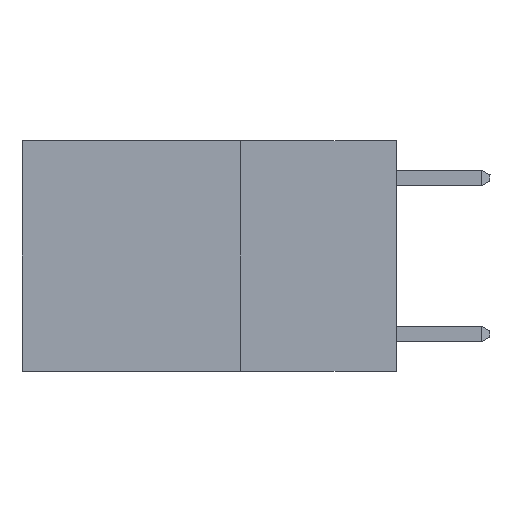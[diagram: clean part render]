
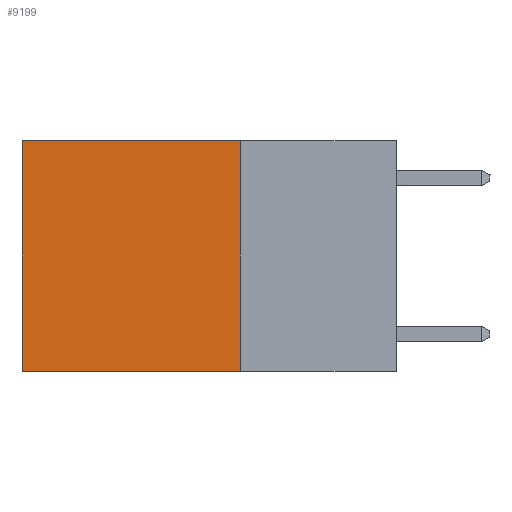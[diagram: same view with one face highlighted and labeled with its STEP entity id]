
A CAD part, left-side view. The second image highlights one B-rep face of the part: STEP entity #9199.
In plain terms, the highlighted planar face has unit normal (-1, 0, 0).
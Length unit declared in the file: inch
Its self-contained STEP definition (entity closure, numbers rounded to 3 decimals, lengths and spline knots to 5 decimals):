
#238 = VERTEX_POINT ( 'NONE', #22340 ) ;
#994 = VERTEX_POINT ( 'NONE', #19007 ) ;
#1125 = LINE ( 'NONE', #6130, #4509 ) ;
#1518 = VECTOR ( 'NONE', #5088, 39.37008 ) ;
#1844 = CARTESIAN_POINT ( 'NONE',  ( 0.2625, 0.6, 0. ) ) ;
#3830 = PLANE ( 'NONE',  #23399 ) ;
#4509 = VECTOR ( 'NONE', #24514, 39.37008 ) ;
#5088 = DIRECTION ( 'NONE',  ( 0., 0., -1. ) ) ;
#5142 = ORIENTED_EDGE ( 'NONE', *, *, #10766, .T. ) ;
#6130 = CARTESIAN_POINT ( 'NONE',  ( 0.2625, 0.25, -0.37 ) ) ;
#8123 = EDGE_LOOP ( 'NONE', ( #5142, #9700, #16774, #9651 ) ) ;
#9199 = ADVANCED_FACE ( 'NONE', ( #30511 ), #3830, .F. ) ;
#9651 = ORIENTED_EDGE ( 'NONE', *, *, #12834, .T. ) ;
#9700 = ORIENTED_EDGE ( 'NONE', *, *, #12046, .F. ) ;
#10766 = EDGE_CURVE ( 'NONE', #20575, #18777, #12174, .T. ) ;
#11542 = CARTESIAN_POINT ( 'NONE',  ( 0.2625, 0.25, 0. ) ) ;
#11650 = CARTESIAN_POINT ( 'NONE',  ( 0.2625, 0.6, 0. ) ) ;
#12046 = EDGE_CURVE ( 'NONE', #994, #18777, #1125, .T. ) ;
#12174 = LINE ( 'NONE', #1844, #23972 ) ;
#12830 = EDGE_CURVE ( 'NONE', #238, #994, #21905, .T. ) ;
#12834 = EDGE_CURVE ( 'NONE', #238, #20575, #16902, .T. ) ;
#13761 = DIRECTION ( 'NONE',  ( 1., 0., 0. ) ) ;
#14233 = CARTESIAN_POINT ( 'NONE',  ( 0.2625, 0.6, -0.37 ) ) ;
#14701 = DIRECTION ( 'NONE',  ( 0., 1., 0. ) ) ;
#16774 = ORIENTED_EDGE ( 'NONE', *, *, #12830, .F. ) ;
#16902 = LINE ( 'NONE', #17051, #24580 ) ;
#17051 = CARTESIAN_POINT ( 'NONE',  ( 0.2625, 0.25, 0. ) ) ;
#18777 = VERTEX_POINT ( 'NONE', #14233 ) ;
#19007 = CARTESIAN_POINT ( 'NONE',  ( 0.2625, 0.25, -0.37 ) ) ;
#19254 = CARTESIAN_POINT ( 'NONE',  ( 0.2625, 0.25, 0. ) ) ;
#20575 = VERTEX_POINT ( 'NONE', #11650 ) ;
#21580 = DIRECTION ( 'NONE',  ( 0., 0., -1. ) ) ;
#21905 = LINE ( 'NONE', #19254, #1518 ) ;
#22340 = CARTESIAN_POINT ( 'NONE',  ( 0.2625, 0.25, 0. ) ) ;
#23399 = AXIS2_PLACEMENT_3D ( 'NONE', #11542, #13761, #28174 ) ;
#23972 = VECTOR ( 'NONE', #21580, 39.37008 ) ;
#24514 = DIRECTION ( 'NONE',  ( 0., 1., 0. ) ) ;
#24580 = VECTOR ( 'NONE', #14701, 39.37008 ) ;
#28174 = DIRECTION ( 'NONE',  ( 0., 0., -1. ) ) ;
#30511 = FACE_OUTER_BOUND ( 'NONE', #8123, .T. ) ;
